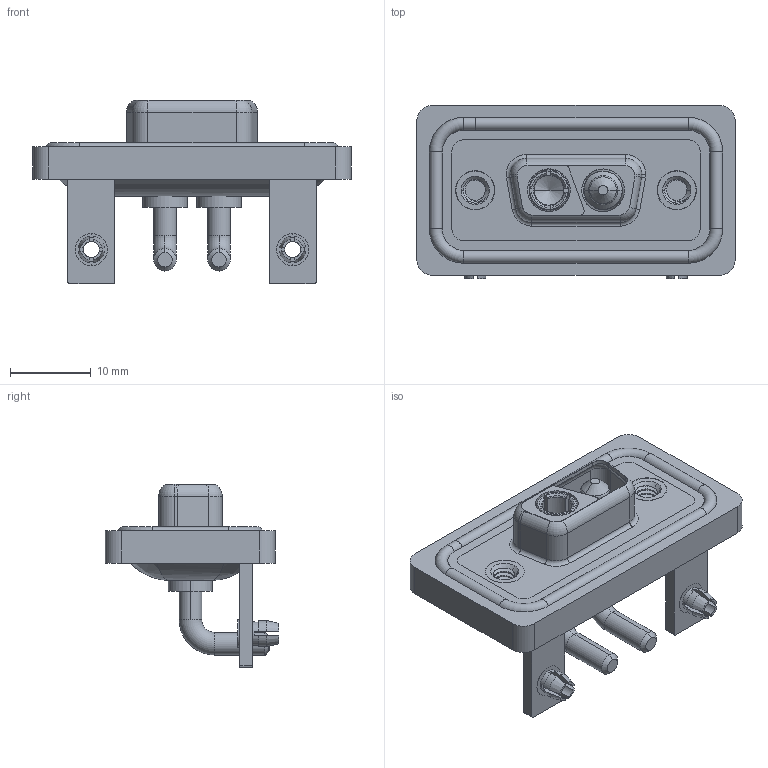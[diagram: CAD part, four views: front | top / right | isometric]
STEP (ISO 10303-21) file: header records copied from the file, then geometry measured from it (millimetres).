
FILE_DESCRIPTION (( 'STEP AP203' ), '1' );
FILE_NAME ('630W2WK2140-2NB.STEP', '2024-04-11T21:22:03', ( '' ), ( '' ), 'SwSTEP 2.0', 'SolidWorks 2023', '' );
FILE_SCHEMA (( 'CONFIG_CONTROL_DESIGN' ));
Length unit declared in the file: millimetre
Products named in the file (10): 630Combo Waterproof Housing_09 Contacts; 630Combo Stabilizer Bracket_50 Contacts; 630Combo Threaded Rivet_A; Power Pin_20A RA; 630Combo Board Lock_50 Contacts; 630Combo Shell Rear_09 Contacts; 630W2WK2140-2NB; Power Socket_20A RA; 630Combo Housing_2WK2; 630Combo Shell Front_09 Contacts
Assembly tree (12 placements, depth 2):
  630W2WK2140-2NB
    630Combo Housing_2WK2
    630Combo Shell Front_09 Contacts
    630Combo Shell Rear_09 Contacts
    630Combo Threaded Rivet_A  x2
    630Combo Stabilizer Bracket_50 Contacts  x2
    630Combo Board Lock_50 Contacts  x2
    Power Socket_20A RA
    Power Pin_20A RA
    630Combo Waterproof Housing_09 Contacts
Bounding box: 39.5 x 21.5 x 22.8 mm (x, y, z)
Volume: 5102 mm3; surface area: 8443.1 mm2
Topology: 15 solids, 15 shells, 642 faces, 1608 edges, 1017 vertices
Faces by surface type: cylinder 289, plane 212, torus 81, cone 48, bspline 12
Entity records: 19293 total; most frequent: CARTESIAN_POINT 5059, DIRECTION 2897, ORIENTED_EDGE 2676, EDGE_CURVE 1338, AXIS2_PLACEMENT_3D 1154, VERTEX_POINT 847, CIRCLE 606, EDGE_LOOP 595
